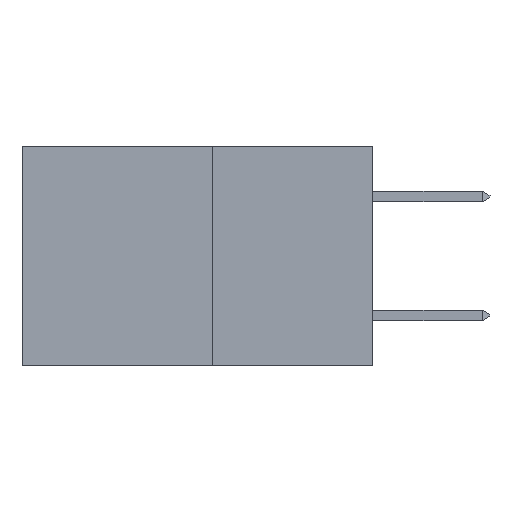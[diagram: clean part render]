
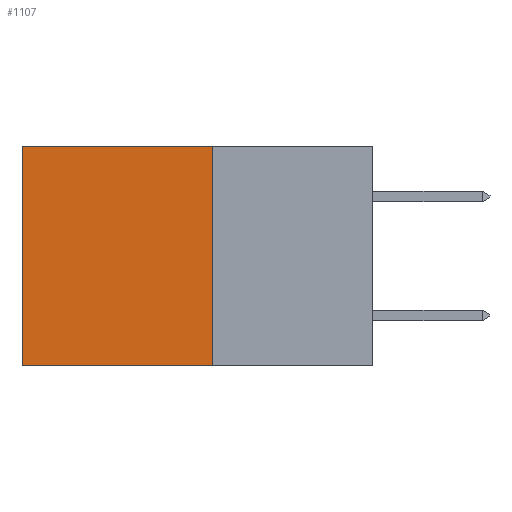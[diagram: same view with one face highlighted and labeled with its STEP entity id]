
A CAD part, left-side view. The second image highlights one B-rep face of the part: STEP entity #1107.
In plain terms, the highlighted planar face has unit normal (-1, 0, 0).
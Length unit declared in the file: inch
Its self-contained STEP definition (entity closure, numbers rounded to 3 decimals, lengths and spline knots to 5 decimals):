
#53 = CARTESIAN_POINT ( 'NONE',  ( 0.277, 0.59, 0. ) ) ;
#217 = VERTEX_POINT ( 'NONE', #53 ) ;
#356 = VERTEX_POINT ( 'NONE', #9795 ) ;
#993 = DIRECTION ( 'NONE',  ( 0., 1., 0. ) ) ;
#1107 = ADVANCED_FACE ( 'NONE', ( #12284 ), #5473, .F. ) ;
#1306 = DIRECTION ( 'NONE',  ( 0., 0., -1. ) ) ;
#1456 = CARTESIAN_POINT ( 'NONE',  ( 0.277, 0.59, -0.37 ) ) ;
#1490 = EDGE_CURVE ( 'NONE', #3547, #356, #2203, .T. ) ;
#2120 = VERTEX_POINT ( 'NONE', #9647 ) ;
#2179 = DIRECTION ( 'NONE',  ( 0., 0., -1. ) ) ;
#2203 = LINE ( 'NONE', #5148, #10283 ) ;
#3299 = CARTESIAN_POINT ( 'NONE',  ( 0.277, 0.27, 0. ) ) ;
#3547 = VERTEX_POINT ( 'NONE', #11217 ) ;
#4072 = EDGE_CURVE ( 'NONE', #2120, #3547, #5983, .T. ) ;
#4713 = LINE ( 'NONE', #3299, #10220 ) ;
#5148 = CARTESIAN_POINT ( 'NONE',  ( 0.277, 0.27, -0.37 ) ) ;
#5149 = EDGE_CURVE ( 'NONE', #217, #356, #13610, .T. ) ;
#5451 = ORIENTED_EDGE ( 'NONE', *, *, #4072, .F. ) ;
#5473 = PLANE ( 'NONE',  #8618 ) ;
#5983 = LINE ( 'NONE', #8737, #13634 ) ;
#6028 = DIRECTION ( 'NONE',  ( 0., 0., -1. ) ) ;
#6146 = EDGE_LOOP ( 'NONE', ( #12880, #10634, #5451, #13446 ) ) ;
#7527 = DIRECTION ( 'NONE',  ( 0., 1., 0. ) ) ;
#8056 = EDGE_CURVE ( 'NONE', #2120, #217, #4713, .T. ) ;
#8204 = DIRECTION ( 'NONE',  ( 1., 0., 0. ) ) ;
#8387 = VECTOR ( 'NONE', #1306, 39.37008 ) ;
#8618 = AXIS2_PLACEMENT_3D ( 'NONE', #11910, #8204, #6028 ) ;
#8737 = CARTESIAN_POINT ( 'NONE',  ( 0.277, 0.27, -0.37 ) ) ;
#9647 = CARTESIAN_POINT ( 'NONE',  ( 0.277, 0.27, 0. ) ) ;
#9795 = CARTESIAN_POINT ( 'NONE',  ( 0.277, 0.59, -0.37 ) ) ;
#10220 = VECTOR ( 'NONE', #7527, 39.37008 ) ;
#10283 = VECTOR ( 'NONE', #993, 39.37008 ) ;
#10634 = ORIENTED_EDGE ( 'NONE', *, *, #1490, .F. ) ;
#11217 = CARTESIAN_POINT ( 'NONE',  ( 0.277, 0.27, -0.37 ) ) ;
#11910 = CARTESIAN_POINT ( 'NONE',  ( 0.277, 0.27, -0.37 ) ) ;
#12284 = FACE_OUTER_BOUND ( 'NONE', #6146, .T. ) ;
#12880 = ORIENTED_EDGE ( 'NONE', *, *, #5149, .T. ) ;
#13446 = ORIENTED_EDGE ( 'NONE', *, *, #8056, .T. ) ;
#13610 = LINE ( 'NONE', #1456, #8387 ) ;
#13634 = VECTOR ( 'NONE', #2179, 39.37008 ) ;
